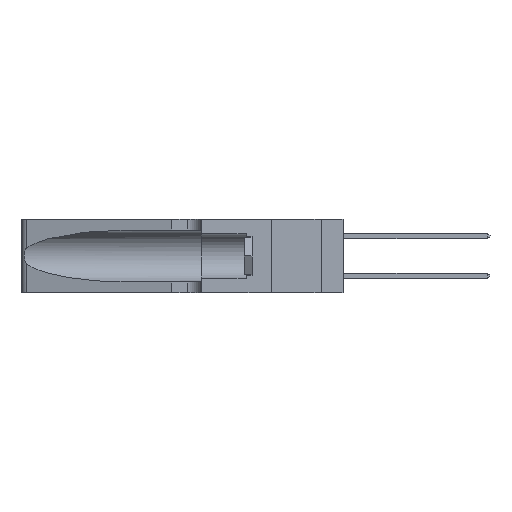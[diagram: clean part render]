
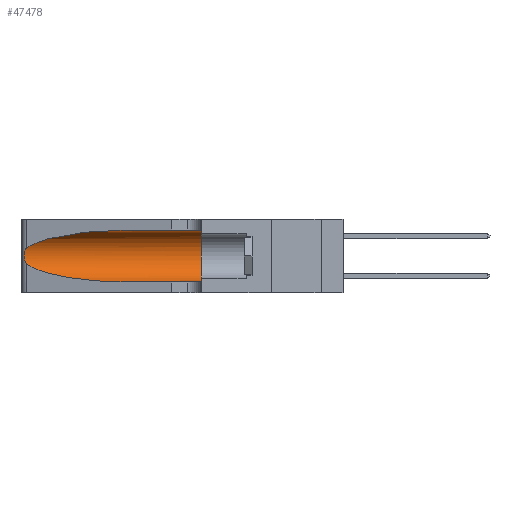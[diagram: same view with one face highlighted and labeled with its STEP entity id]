
A CAD part, left-side view. The second image highlights one B-rep face of the part: STEP entity #47478.
In plain terms, the highlighted cylindrical face has radius 3.308 mm (diameter 6.617 mm), a partial arc.
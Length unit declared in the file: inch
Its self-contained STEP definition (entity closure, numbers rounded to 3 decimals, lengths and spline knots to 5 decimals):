
#73 = CARTESIAN_POINT ( 'NONE',  ( 0.25555, 1.22993, 0.14849 ) ) ;
#1172 = CARTESIAN_POINT ( 'NONE',  ( 0.18966, 0.96281, 0.31525 ) ) ;
#1326 = CARTESIAN_POINT ( 'NONE',  ( 0.1305, 0.72297, 0.05475 ) ) ;
#1515 = CARTESIAN_POINT ( 'NONE',  ( 0.1305, 0.35, 0.185 ) ) ;
#2049 = CARTESIAN_POINT ( 'NONE',  ( 0.25487, 1.22718, 0.14631 ) ) ;
#2215 = VERTEX_POINT ( 'NONE', #36666 ) ;
#2332 = CARTESIAN_POINT ( 'NONE',  ( 0.25487, 1.22718, 0.22369 ) ) ;
#2793 = CARTESIAN_POINT ( 'NONE',  ( 0.1305, 1.61858, 0.31525 ) ) ;
#3310 = CIRCLE ( 'NONE', #5370, 0.13025 ) ;
#3598 = CARTESIAN_POINT ( 'NONE',  ( 0.25639, 1.23184, 0.21858 ) ) ;
#4931 =( BOUNDED_CURVE ( )  B_SPLINE_CURVE ( 3, ( #2049, #38595, #27540, #7781 ),
 .UNSPECIFIED., .F., .F. ) 
 B_SPLINE_CURVE_WITH_KNOTS ( ( 4, 4 ),
 ( 3.44316, 4.71239 ),
 .UNSPECIFIED. ) 
 CURVE ( )  GEOMETRIC_REPRESENTATION_ITEM ( )  RATIONAL_B_SPLINE_CURVE ( ( 1., 0.87, 0.87, 1. ) ) 
 REPRESENTATION_ITEM ( '' )  );
#5262 = VECTOR ( 'NONE', #38987, 39.37008 ) ;
#5370 = AXIS2_PLACEMENT_3D ( 'NONE', #1515, #17138, #33084 ) ;
#6868 = VERTEX_POINT ( 'NONE', #1326 ) ;
#6890 = ORIENTED_EDGE ( 'NONE', *, *, #19280, .T. ) ;
#7192 = DIRECTION ( 'NONE',  ( 0., -1., 0. ) ) ;
#7704 = CARTESIAN_POINT ( 'NONE',  ( 0.1305, 1.61858, 0.185 ) ) ;
#7781 = CARTESIAN_POINT ( 'NONE',  ( 0.1305, 0.72297, 0.05475 ) ) ;
#8197 = EDGE_CURVE ( 'NONE', #20174, #6868, #4931, .T. ) ;
#8485 = VERTEX_POINT ( 'NONE', #2332 ) ;
#8759 = B_SPLINE_CURVE_WITH_KNOTS ( 'NONE', 3,
 ( #23394, #27377, #3598, #47402, #31831, #12448, #20758, #40089, #36135, #16219, #24392, #12271, #73, #31998 ),
 .UNSPECIFIED., .F., .F.,
 ( 4, 2, 2, 2, 2, 2, 4 ),
 ( 0., 0.00027, 0.00053, 0.00107, 0.0016, 0.00187, 0.00214 ),
 .UNSPECIFIED. ) ;
#9197 = CARTESIAN_POINT ( 'NONE',  ( 0.25487, 1.22718, 0.22369 ) ) ;
#9465 = ORIENTED_EDGE ( 'NONE', *, *, #40289, .T. ) ;
#12271 = CARTESIAN_POINT ( 'NONE',  ( 0.25639, 1.23186, 0.15144 ) ) ;
#12448 = CARTESIAN_POINT ( 'NONE',  ( 0.26018, 1.23835, 0.19895 ) ) ;
#15792 = VERTEX_POINT ( 'NONE', #50455 ) ;
#16219 = CARTESIAN_POINT ( 'NONE',  ( 0.25856, 1.23593, 0.16098 ) ) ;
#16543 = CARTESIAN_POINT ( 'NONE',  ( 0.1305, 0.35, 0.05475 ) ) ;
#17138 = DIRECTION ( 'NONE',  ( 0., 1., 0. ) ) ;
#19280 = EDGE_CURVE ( 'NONE', #15792, #8485, #36355, .T. ) ;
#20066 = AXIS2_PLACEMENT_3D ( 'NONE', #7704, #7192, #47165 ) ;
#20174 = VERTEX_POINT ( 'NONE', #22293 ) ;
#20758 = CARTESIAN_POINT ( 'NONE',  ( 0.26075, 1.23896, 0.19203 ) ) ;
#21312 = CARTESIAN_POINT ( 'NONE',  ( 0.2373, 1.15595, 0.28018 ) ) ;
#22293 = CARTESIAN_POINT ( 'NONE',  ( 0.25487, 1.22718, 0.14631 ) ) ;
#23011 = CARTESIAN_POINT ( 'NONE',  ( 0.1305, 1.61858, 0.05475 ) ) ;
#23394 = CARTESIAN_POINT ( 'NONE',  ( 0.25487, 1.22718, 0.22369 ) ) ;
#24392 = CARTESIAN_POINT ( 'NONE',  ( 0.25789, 1.23486, 0.15765 ) ) ;
#24521 = EDGE_CURVE ( 'NONE', #2215, #44421, #3310, .T. ) ;
#27377 = CARTESIAN_POINT ( 'NONE',  ( 0.25555, 1.22994, 0.2215 ) ) ;
#27540 = CARTESIAN_POINT ( 'NONE',  ( 0.18966, 0.96281, 0.05475 ) ) ;
#28177 = ORIENTED_EDGE ( 'NONE', *, *, #24521, .F. ) ;
#29115 = CYLINDRICAL_SURFACE ( 'NONE', #20066, 0.13025 ) ;
#29544 = EDGE_CURVE ( 'NONE', #15792, #2215, #41203, .T. ) ;
#30330 = FACE_OUTER_BOUND ( 'NONE', #44030, .T. ) ;
#31518 = LINE ( 'NONE', #23011, #45771 ) ;
#31831 = CARTESIAN_POINT ( 'NONE',  ( 0.25854, 1.2359, 0.20912 ) ) ;
#31998 = CARTESIAN_POINT ( 'NONE',  ( 0.25487, 1.22718, 0.14631 ) ) ;
#33084 = DIRECTION ( 'NONE',  ( 0., 0., 1. ) ) ;
#36135 = CARTESIAN_POINT ( 'NONE',  ( 0.26017, 1.23833, 0.17102 ) ) ;
#36355 =( BOUNDED_CURVE ( )  B_SPLINE_CURVE ( 3, ( #37238, #1172, #21312, #9197 ),
 .UNSPECIFIED., .F., .T. ) 
 B_SPLINE_CURVE_WITH_KNOTS ( ( 4, 4 ),
 ( 1.5708, 2.84003 ),
 .UNSPECIFIED. ) 
 CURVE ( )  GEOMETRIC_REPRESENTATION_ITEM ( )  RATIONAL_B_SPLINE_CURVE ( ( 1., 0.87, 0.87, 1. ) ) 
 REPRESENTATION_ITEM ( '' )  );
#36444 = EDGE_CURVE ( 'NONE', #8485, #20174, #8759, .T. ) ;
#36666 = CARTESIAN_POINT ( 'NONE',  ( 0.1305, 0.35, 0.31525 ) ) ;
#37238 = CARTESIAN_POINT ( 'NONE',  ( 0.1305, 0.72297, 0.31525 ) ) ;
#38595 = CARTESIAN_POINT ( 'NONE',  ( 0.2373, 1.15595, 0.08982 ) ) ;
#38987 = DIRECTION ( 'NONE',  ( 0., -1., 0. ) ) ;
#39455 = ORIENTED_EDGE ( 'NONE', *, *, #8197, .T. ) ;
#40089 = CARTESIAN_POINT ( 'NONE',  ( 0.26075, 1.23896, 0.178 ) ) ;
#40289 = EDGE_CURVE ( 'NONE', #6868, #44421, #31518, .T. ) ;
#41203 = LINE ( 'NONE', #2793, #5262 ) ;
#44030 = EDGE_LOOP ( 'NONE', ( #6890, #45842, #39455, #9465, #28177, #49390 ) ) ;
#44421 = VERTEX_POINT ( 'NONE', #16543 ) ;
#45771 = VECTOR ( 'NONE', #46871, 39.37008 ) ;
#45842 = ORIENTED_EDGE ( 'NONE', *, *, #36444, .T. ) ;
#46871 = DIRECTION ( 'NONE',  ( 0., -1., 0. ) ) ;
#47165 = DIRECTION ( 'NONE',  ( 0., 0., -1. ) ) ;
#47402 = CARTESIAN_POINT ( 'NONE',  ( 0.25787, 1.23484, 0.2124 ) ) ;
#47478 = ADVANCED_FACE ( 'NONE', ( #30330 ), #29115, .F. ) ;
#49390 = ORIENTED_EDGE ( 'NONE', *, *, #29544, .F. ) ;
#50455 = CARTESIAN_POINT ( 'NONE',  ( 0.1305, 0.72297, 0.31525 ) ) ;
